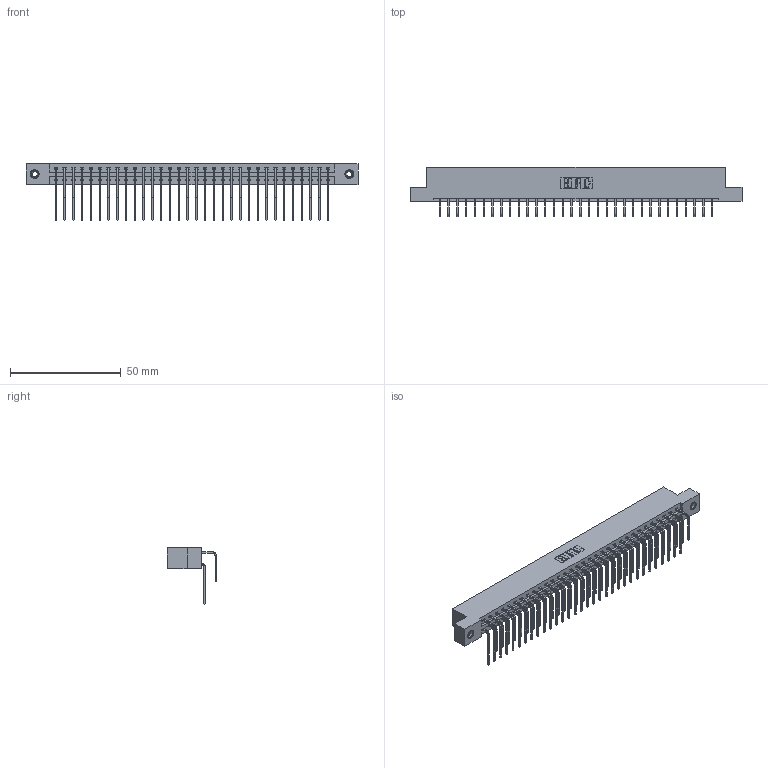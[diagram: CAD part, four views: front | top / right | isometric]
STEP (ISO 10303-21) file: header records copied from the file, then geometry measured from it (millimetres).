
FILE_DESCRIPTION (( 'STEP AP203' ), '1' );
FILE_NAME ('337-064-558-208.STEP', '2018-08-11T06:40:53', ( '' ), ( '' ), 'SwSTEP 2.0', 'SolidWorks 2016', '' );
FILE_SCHEMA (( 'CONFIG_CONTROL_DESIGN' ));
Length unit declared in the file: inch
Products named in the file (5): 345-292-001_558 559 Tail - 1; 345-292-001_558 Tail - 2; 345-250-001_345-250-003-102; 337-064-558-208; 337 Part_Flush Mounting Lugs - 0.156 Dia-TI
Assembly tree (67 placements, depth 2):
  337-064-558-208
    337 Part_Flush Mounting Lugs - 0.156 Dia-TI
    345-292-001_558 559 Tail - 1  x32
    345-292-001_558 Tail - 2  x32
    345-250-001_345-250-003-102  x2
Bounding box: 149.81 x 22.17 x 25.53 mm (x, y, z)
Volume: 16017.7 mm3; surface area: 19888.6 mm2
Topology: 67 solids, 67 shells, 3758 faces, 11135 edges, 7330 vertices
Faces by surface type: plane 2662, cylinder 1080, cone 12, torus 4
Entity records: 29074 total; most frequent: CARTESIAN_POINT 4932, ORIENTED_EDGE 4810, DIRECTION 4227, EDGE_CURVE 2405, LINE 2217, VECTOR 2217, VERTEX_POINT 1596, AXIS2_PLACEMENT_3D 1005
